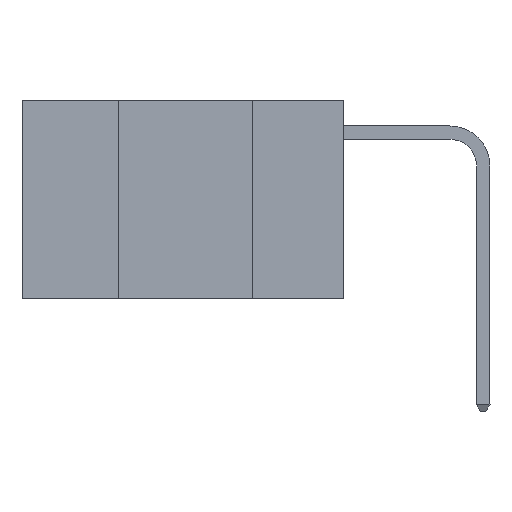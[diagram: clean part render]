
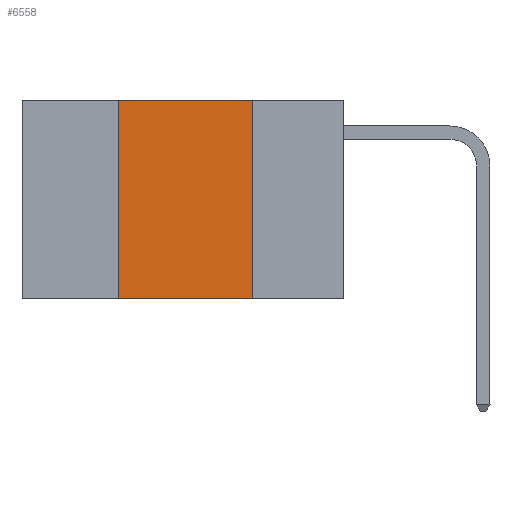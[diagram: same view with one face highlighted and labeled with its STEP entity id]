
A CAD part, left-side view. The second image highlights one B-rep face of the part: STEP entity #6558.
In plain terms, the highlighted planar face has unit normal (-1, 0, 0).
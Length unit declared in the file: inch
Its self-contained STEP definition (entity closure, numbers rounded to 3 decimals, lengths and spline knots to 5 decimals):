
#49 = FACE_OUTER_BOUND ( 'NONE', #7120, .T. ) ;
#823 = CARTESIAN_POINT ( 'NONE',  ( 0., 0.6, 0. ) ) ;
#908 = DIRECTION ( 'NONE',  ( 0., 0., -1. ) ) ;
#1477 = VERTEX_POINT ( 'NONE', #13294 ) ;
#2317 = LINE ( 'NONE', #9349, #11875 ) ;
#3406 = VERTEX_POINT ( 'NONE', #4470 ) ;
#3886 = VECTOR ( 'NONE', #908, 39.37008 ) ;
#4470 = CARTESIAN_POINT ( 'NONE',  ( 0., 0.17, -0.37 ) ) ;
#4812 = DIRECTION ( 'NONE',  ( 0., -1., 0. ) ) ;
#4910 = LINE ( 'NONE', #13920, #7905 ) ;
#6008 = DIRECTION ( 'NONE',  ( 1., 0., 0. ) ) ;
#6192 = VERTEX_POINT ( 'NONE', #15274 ) ;
#6382 = VERTEX_POINT ( 'NONE', #13102 ) ;
#6558 = ADVANCED_FACE ( 'NONE', ( #49 ), #13446, .F. ) ;
#6890 = DIRECTION ( 'NONE',  ( 0., -1., 0. ) ) ;
#7120 = EDGE_LOOP ( 'NONE', ( #10430, #10445, #10524, #10594 ) ) ;
#7905 = VECTOR ( 'NONE', #15169, 39.37008 ) ;
#8002 = EDGE_CURVE ( 'NONE', #6192, #3406, #2317, .T. ) ;
#8399 = AXIS2_PLACEMENT_3D ( 'NONE', #823, #6008, #14728 ) ;
#9349 = CARTESIAN_POINT ( 'NONE',  ( 0., 0.6, -0.37 ) ) ;
#9670 = CARTESIAN_POINT ( 'NONE',  ( 0., 0.17, 0. ) ) ;
#10398 = EDGE_CURVE ( 'NONE', #6192, #6382, #4910, .T. ) ;
#10430 = ORIENTED_EDGE ( 'NONE', *, *, #12087, .F. ) ;
#10445 = ORIENTED_EDGE ( 'NONE', *, *, #13731, .F. ) ;
#10524 = ORIENTED_EDGE ( 'NONE', *, *, #10398, .F. ) ;
#10594 = ORIENTED_EDGE ( 'NONE', *, *, #8002, .T. ) ;
#11183 = VECTOR ( 'NONE', #4812, 39.37008 ) ;
#11875 = VECTOR ( 'NONE', #6890, 39.37008 ) ;
#12087 = EDGE_CURVE ( 'NONE', #1477, #3406, #14272, .T. ) ;
#13102 = CARTESIAN_POINT ( 'NONE',  ( 0., 0.42, 0. ) ) ;
#13294 = CARTESIAN_POINT ( 'NONE',  ( 0., 0.17, 0. ) ) ;
#13446 = PLANE ( 'NONE',  #8399 ) ;
#13571 = CARTESIAN_POINT ( 'NONE',  ( 0., 0.6, 0. ) ) ;
#13731 = EDGE_CURVE ( 'NONE', #6382, #1477, #14993, .T. ) ;
#13920 = CARTESIAN_POINT ( 'NONE',  ( 0., 0.42, 0. ) ) ;
#14272 = LINE ( 'NONE', #9670, #3886 ) ;
#14728 = DIRECTION ( 'NONE',  ( 0., 0., -1. ) ) ;
#14993 = LINE ( 'NONE', #13571, #11183 ) ;
#15169 = DIRECTION ( 'NONE',  ( 0., 0., 1. ) ) ;
#15274 = CARTESIAN_POINT ( 'NONE',  ( 0., 0.42, -0.37 ) ) ;
